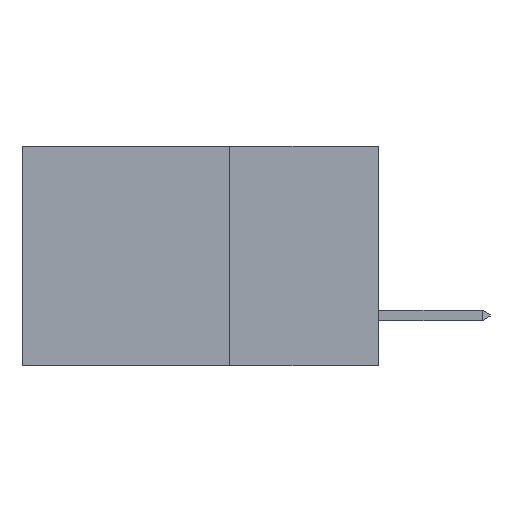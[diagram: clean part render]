
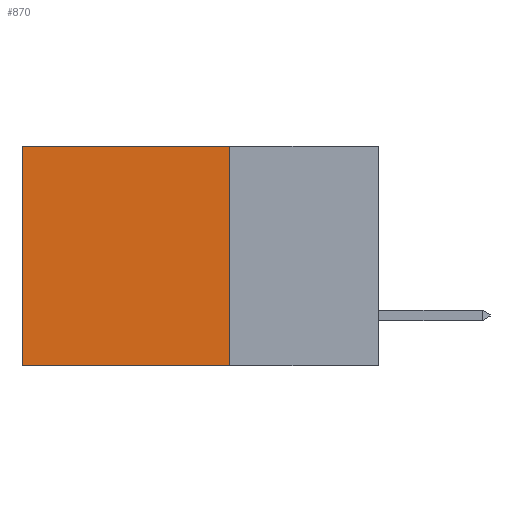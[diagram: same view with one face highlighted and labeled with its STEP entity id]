
A CAD part, left-side view. The second image highlights one B-rep face of the part: STEP entity #870.
In plain terms, the highlighted planar face has unit normal (-1, 0, 0).
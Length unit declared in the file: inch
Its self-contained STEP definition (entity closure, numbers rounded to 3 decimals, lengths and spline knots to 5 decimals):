
#115 = CARTESIAN_POINT ( 'NONE',  ( 0.298, 0.25, 0. ) ) ;
#527 = CARTESIAN_POINT ( 'NONE',  ( 0.298, 0.6, 0. ) ) ;
#754 = AXIS2_PLACEMENT_3D ( 'NONE', #115, #9445, #9432 ) ;
#762 = VERTEX_POINT ( 'NONE', #1598 ) ;
#870 = ADVANCED_FACE ( 'NONE', ( #10881 ), #8517, .F. ) ;
#1031 = CARTESIAN_POINT ( 'NONE',  ( 0.298, 0.25, 0. ) ) ;
#1598 = CARTESIAN_POINT ( 'NONE',  ( 0.298, 0.6, 0. ) ) ;
#2073 = EDGE_CURVE ( 'NONE', #762, #4753, #8455, .T. ) ;
#2258 = DIRECTION ( 'NONE',  ( 0., 0., -1. ) ) ;
#2360 = ORIENTED_EDGE ( 'NONE', *, *, #2073, .T. ) ;
#2616 = VECTOR ( 'NONE', #12183, 39.37008 ) ;
#2860 = VECTOR ( 'NONE', #2258, 39.37008 ) ;
#3036 = DIRECTION ( 'NONE',  ( 0., 1., 0. ) ) ;
#4633 = CARTESIAN_POINT ( 'NONE',  ( 0.298, 0.6, -0.37 ) ) ;
#4753 = VERTEX_POINT ( 'NONE', #4633 ) ;
#5067 = ORIENTED_EDGE ( 'NONE', *, *, #11043, .F. ) ;
#5882 = EDGE_CURVE ( 'NONE', #13462, #10425, #10918, .T. ) ;
#6196 = CARTESIAN_POINT ( 'NONE',  ( 0.298, 0.25, -0.37 ) ) ;
#8042 = ORIENTED_EDGE ( 'NONE', *, *, #5882, .F. ) ;
#8455 = LINE ( 'NONE', #527, #2616 ) ;
#8517 = PLANE ( 'NONE',  #754 ) ;
#8544 = LINE ( 'NONE', #13761, #11109 ) ;
#9129 = ORIENTED_EDGE ( 'NONE', *, *, #9339, .T. ) ;
#9339 = EDGE_CURVE ( 'NONE', #13462, #762, #9982, .T. ) ;
#9432 = DIRECTION ( 'NONE',  ( 0., 0., -1. ) ) ;
#9445 = DIRECTION ( 'NONE',  ( 1., 0., 0. ) ) ;
#9597 = CARTESIAN_POINT ( 'NONE',  ( 0.298, 0.25, 0. ) ) ;
#9982 = LINE ( 'NONE', #9597, #12857 ) ;
#10425 = VERTEX_POINT ( 'NONE', #6196 ) ;
#10545 = DIRECTION ( 'NONE',  ( 0., 1., 0. ) ) ;
#10881 = FACE_OUTER_BOUND ( 'NONE', #12791, .T. ) ;
#10918 = LINE ( 'NONE', #1031, #2860 ) ;
#11043 = EDGE_CURVE ( 'NONE', #10425, #4753, #8544, .T. ) ;
#11109 = VECTOR ( 'NONE', #10545, 39.37008 ) ;
#11455 = CARTESIAN_POINT ( 'NONE',  ( 0.298, 0.25, 0. ) ) ;
#12183 = DIRECTION ( 'NONE',  ( 0., 0., -1. ) ) ;
#12791 = EDGE_LOOP ( 'NONE', ( #2360, #5067, #8042, #9129 ) ) ;
#12857 = VECTOR ( 'NONE', #3036, 39.37008 ) ;
#13462 = VERTEX_POINT ( 'NONE', #11455 ) ;
#13761 = CARTESIAN_POINT ( 'NONE',  ( 0.298, 0.25, -0.37 ) ) ;
